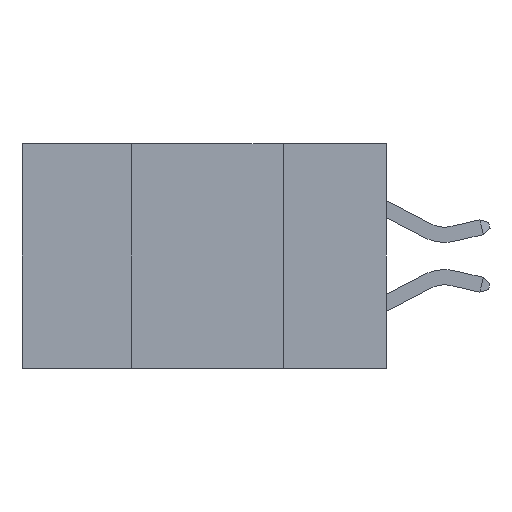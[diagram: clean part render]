
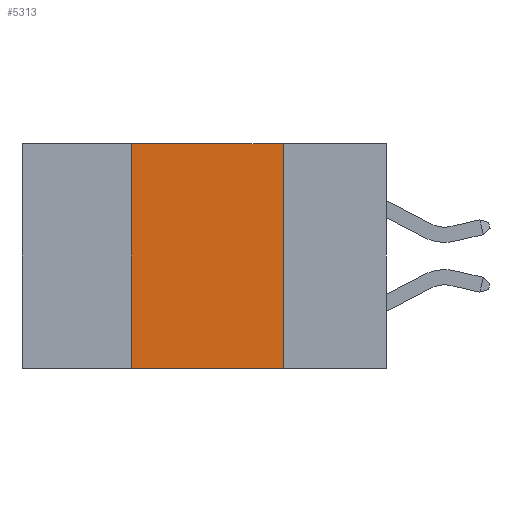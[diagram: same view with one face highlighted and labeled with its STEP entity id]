
A CAD part, left-side view. The second image highlights one B-rep face of the part: STEP entity #5313.
In plain terms, the highlighted planar face has unit normal (-1, 0, 0).
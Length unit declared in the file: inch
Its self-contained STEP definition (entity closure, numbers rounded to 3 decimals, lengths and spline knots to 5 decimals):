
#764 = DIRECTION ( 'NONE',  ( 0., 0., 1. ) ) ;
#1354 = DIRECTION ( 'NONE',  ( 0., -1., 0. ) ) ;
#1512 = CARTESIAN_POINT ( 'NONE',  ( 0., 0.42, 0. ) ) ;
#1893 = DIRECTION ( 'NONE',  ( 0., 0., -1. ) ) ;
#1912 = CARTESIAN_POINT ( 'NONE',  ( 0., 0.17, -0.37 ) ) ;
#2162 = FACE_OUTER_BOUND ( 'NONE', #6928, .T. ) ;
#3405 = VECTOR ( 'NONE', #764, 39.37008 ) ;
#3590 = DIRECTION ( 'NONE',  ( 0., -1., 0. ) ) ;
#3686 = AXIS2_PLACEMENT_3D ( 'NONE', #8144, #11106, #1893 ) ;
#3698 = VECTOR ( 'NONE', #9376, 39.37008 ) ;
#4128 = CARTESIAN_POINT ( 'NONE',  ( 0., 0.17, -0.37 ) ) ;
#4174 = EDGE_CURVE ( 'NONE', #4501, #12842, #10647, .T. ) ;
#4501 = VERTEX_POINT ( 'NONE', #7530 ) ;
#4531 = LINE ( 'NONE', #6377, #6423 ) ;
#4640 = ORIENTED_EDGE ( 'NONE', *, *, #10792, .F. ) ;
#5313 = ADVANCED_FACE ( 'NONE', ( #2162 ), #8205, .F. ) ;
#5489 = LINE ( 'NONE', #11479, #12069 ) ;
#6057 = VERTEX_POINT ( 'NONE', #1912 ) ;
#6377 = CARTESIAN_POINT ( 'NONE',  ( 0., 0.6, 0. ) ) ;
#6423 = VECTOR ( 'NONE', #1354, 39.37008 ) ;
#6928 = EDGE_LOOP ( 'NONE', ( #4640, #8490, #8327, #7135 ) ) ;
#7135 = ORIENTED_EDGE ( 'NONE', *, *, #9658, .T. ) ;
#7530 = CARTESIAN_POINT ( 'NONE',  ( 0., 0.42, -0.37 ) ) ;
#8144 = CARTESIAN_POINT ( 'NONE',  ( 0., 0.6, 0. ) ) ;
#8205 = PLANE ( 'NONE',  #3686 ) ;
#8297 = VERTEX_POINT ( 'NONE', #12482 ) ;
#8327 = ORIENTED_EDGE ( 'NONE', *, *, #4174, .F. ) ;
#8490 = ORIENTED_EDGE ( 'NONE', *, *, #12351, .F. ) ;
#9376 = DIRECTION ( 'NONE',  ( 0., 0., -1. ) ) ;
#9658 = EDGE_CURVE ( 'NONE', #4501, #6057, #5489, .T. ) ;
#10647 = LINE ( 'NONE', #12682, #3405 ) ;
#10792 = EDGE_CURVE ( 'NONE', #8297, #6057, #12203, .T. ) ;
#11106 = DIRECTION ( 'NONE',  ( 1., 0., 0. ) ) ;
#11479 = CARTESIAN_POINT ( 'NONE',  ( 0., 0.6, -0.37 ) ) ;
#12069 = VECTOR ( 'NONE', #3590, 39.37008 ) ;
#12203 = LINE ( 'NONE', #4128, #3698 ) ;
#12351 = EDGE_CURVE ( 'NONE', #12842, #8297, #4531, .T. ) ;
#12482 = CARTESIAN_POINT ( 'NONE',  ( 0., 0.17, 0. ) ) ;
#12682 = CARTESIAN_POINT ( 'NONE',  ( 0., 0.42, -0.37 ) ) ;
#12842 = VERTEX_POINT ( 'NONE', #1512 ) ;
